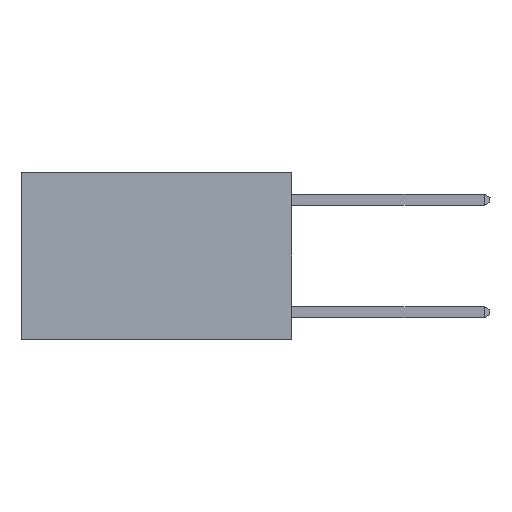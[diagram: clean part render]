
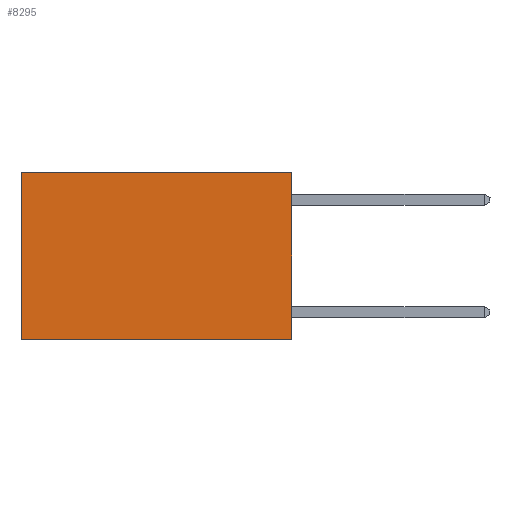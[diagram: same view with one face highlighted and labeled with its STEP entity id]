
A CAD part, left-side view. The second image highlights one B-rep face of the part: STEP entity #8295.
In plain terms, the highlighted planar face has unit normal (-1, 0, 0).
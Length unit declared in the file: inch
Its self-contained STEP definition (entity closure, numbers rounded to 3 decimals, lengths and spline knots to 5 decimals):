
#1290 = VERTEX_POINT ( 'NONE', #11405 ) ;
#1391 = CARTESIAN_POINT ( 'NONE',  ( 0.2625, 0.6, 0. ) ) ;
#1893 = VECTOR ( 'NONE', #14516, 39.37008 ) ;
#3125 = EDGE_CURVE ( 'NONE', #1290, #10542, #4154, .T. ) ;
#3179 = DIRECTION ( 'NONE',  ( 0., 0., -1. ) ) ;
#3437 = CARTESIAN_POINT ( 'NONE',  ( 0.2625, 0.6, 0. ) ) ;
#3749 = ORIENTED_EDGE ( 'NONE', *, *, #12465, .T. ) ;
#3766 = AXIS2_PLACEMENT_3D ( 'NONE', #11645, #11856, #7402 ) ;
#4015 = CARTESIAN_POINT ( 'NONE',  ( 0.2625, 0., -0.37 ) ) ;
#4095 = DIRECTION ( 'NONE',  ( 0., 1., 0. ) ) ;
#4154 = LINE ( 'NONE', #11088, #1893 ) ;
#4325 = EDGE_CURVE ( 'NONE', #8133, #11805, #6311, .T. ) ;
#4758 = CARTESIAN_POINT ( 'NONE',  ( 0.2625, 0.6, -0.37 ) ) ;
#4846 = ORIENTED_EDGE ( 'NONE', *, *, #3125, .T. ) ;
#4885 = FACE_OUTER_BOUND ( 'NONE', #11258, .T. ) ;
#6118 = ORIENTED_EDGE ( 'NONE', *, *, #13574, .F. ) ;
#6193 = PLANE ( 'NONE',  #3766 ) ;
#6311 = LINE ( 'NONE', #4015, #8718 ) ;
#7402 = DIRECTION ( 'NONE',  ( 0., 0., -1. ) ) ;
#8133 = VERTEX_POINT ( 'NONE', #13645 ) ;
#8179 = VECTOR ( 'NONE', #3179, 39.37008 ) ;
#8295 = ADVANCED_FACE ( 'NONE', ( #4885 ), #6193, .F. ) ;
#8718 = VECTOR ( 'NONE', #4095, 39.37008 ) ;
#8888 = LINE ( 'NONE', #10050, #8179 ) ;
#10050 = CARTESIAN_POINT ( 'NONE',  ( 0.2625, 0., 0. ) ) ;
#10542 = VERTEX_POINT ( 'NONE', #1391 ) ;
#11088 = CARTESIAN_POINT ( 'NONE',  ( 0.2625, 0., 0. ) ) ;
#11258 = EDGE_LOOP ( 'NONE', ( #3749, #11527, #6118, #4846 ) ) ;
#11265 = LINE ( 'NONE', #3437, #14274 ) ;
#11405 = CARTESIAN_POINT ( 'NONE',  ( 0.2625, 0., 0. ) ) ;
#11527 = ORIENTED_EDGE ( 'NONE', *, *, #4325, .F. ) ;
#11645 = CARTESIAN_POINT ( 'NONE',  ( 0.2625, 0., 0. ) ) ;
#11805 = VERTEX_POINT ( 'NONE', #4758 ) ;
#11856 = DIRECTION ( 'NONE',  ( 1., 0., 0. ) ) ;
#12465 = EDGE_CURVE ( 'NONE', #10542, #11805, #11265, .T. ) ;
#13574 = EDGE_CURVE ( 'NONE', #1290, #8133, #8888, .T. ) ;
#13645 = CARTESIAN_POINT ( 'NONE',  ( 0.2625, 0., -0.37 ) ) ;
#13773 = DIRECTION ( 'NONE',  ( 0., 0., -1. ) ) ;
#14274 = VECTOR ( 'NONE', #13773, 39.37008 ) ;
#14516 = DIRECTION ( 'NONE',  ( 0., 1., 0. ) ) ;
